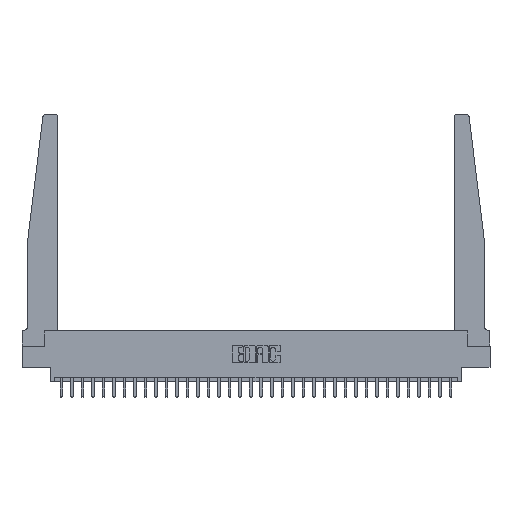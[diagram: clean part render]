
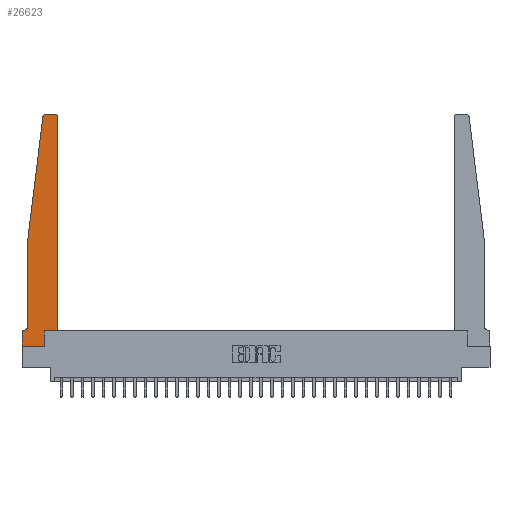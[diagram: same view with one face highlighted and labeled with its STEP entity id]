
A CAD part, top view. The second image highlights one B-rep face of the part: STEP entity #26623.
In plain terms, the highlighted planar face has unit normal (0, 0, 1).
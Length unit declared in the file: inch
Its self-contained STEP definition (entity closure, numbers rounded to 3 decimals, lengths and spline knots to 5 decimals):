
#387 = ORIENTED_EDGE ( 'NONE', *, *, #27444, .T. ) ;
#1822 = VECTOR ( 'NONE', #2126, 39.37008 ) ;
#1898 = CARTESIAN_POINT ( 'NONE',  ( 0.27653, 2.72, 0.37 ) ) ;
#2126 = DIRECTION ( 'NONE',  ( -1., 0., 0. ) ) ;
#2242 = CARTESIAN_POINT ( 'NONE',  ( 0.25, 2.75, 0.37 ) ) ;
#2247 = DIRECTION ( 'NONE',  ( 0., 1., 0. ) ) ;
#2527 = EDGE_CURVE ( 'NONE', #8599, #23406, #13665, .T. ) ;
#2587 = LINE ( 'NONE', #27826, #1822 ) ;
#2915 = EDGE_CURVE ( 'NONE', #23406, #12471, #2587, .T. ) ;
#3376 = VERTEX_POINT ( 'NONE', #18267 ) ;
#4134 = PLANE ( 'NONE',  #16970 ) ;
#4220 = VECTOR ( 'NONE', #27223, 39.37008 ) ;
#4279 = DIRECTION ( 'NONE',  ( 1., 0., 0. ) ) ;
#4394 = DIRECTION ( 'NONE',  ( -0.122, -0.992, 0. ) ) ;
#5062 = LINE ( 'NONE', #23875, #29171 ) ;
#6013 = VERTEX_POINT ( 'NONE', #14080 ) ;
#6069 = VECTOR ( 'NONE', #4394, 39.37008 ) ;
#6763 = AXIS2_PLACEMENT_3D ( 'NONE', #26341, #12355, #28664 ) ;
#6806 = LINE ( 'NONE', #27824, #6069 ) ;
#7369 = VERTEX_POINT ( 'NONE', #12664 ) ;
#7890 = CARTESIAN_POINT ( 'NONE',  ( 0., 0.1875, 0.37 ) ) ;
#8506 = ORIENTED_EDGE ( 'NONE', *, *, #21793, .T. ) ;
#8599 = VERTEX_POINT ( 'NONE', #24033 ) ;
#9480 = CARTESIAN_POINT ( 'NONE',  ( 0.395, 2.72, 0.37 ) ) ;
#10293 = CARTESIAN_POINT ( 'NONE',  ( 0.015, 0.1875, 0.37 ) ) ;
#10484 = EDGE_CURVE ( 'NONE', #17360, #7369, #5062, .T. ) ;
#10695 = AXIS2_PLACEMENT_3D ( 'NONE', #1898, #18375, #4279 ) ;
#10699 = CARTESIAN_POINT ( 'NONE',  ( 0.395, 2.75, 0.37 ) ) ;
#10746 = ORIENTED_EDGE ( 'NONE', *, *, #30219, .T. ) ;
#10862 = CARTESIAN_POINT ( 'NONE',  ( 0.065, 1.25, 0.37 ) ) ;
#11195 = CARTESIAN_POINT ( 'NONE',  ( 0., 0.1875, 0.37 ) ) ;
#11690 = CARTESIAN_POINT ( 'NONE',  ( 0.425, 0.18, 0.37 ) ) ;
#11843 = DIRECTION ( 'NONE',  ( 1., 0., 0. ) ) ;
#12089 = CARTESIAN_POINT ( 'NONE',  ( 0., 0., 0.37 ) ) ;
#12327 = VECTOR ( 'NONE', #2247, 39.37008 ) ;
#12355 = DIRECTION ( 'NONE',  ( 0., 0., -1. ) ) ;
#12471 = VERTEX_POINT ( 'NONE', #7890 ) ;
#12664 = CARTESIAN_POINT ( 'NONE',  ( 0.2605, 0., 0.37 ) ) ;
#13452 = CARTESIAN_POINT ( 'NONE',  ( 0.2605, 0.18, 0.37 ) ) ;
#13602 = DIRECTION ( 'NONE',  ( 1., 0., 0. ) ) ;
#13665 = CIRCLE ( 'NONE', #6763, 0.05 ) ;
#13998 = CARTESIAN_POINT ( 'NONE',  ( 0.2605, 0.18, 0.37 ) ) ;
#14019 = CARTESIAN_POINT ( 'NONE',  ( 0.425, 0.18, 0.37 ) ) ;
#14080 = CARTESIAN_POINT ( 'NONE',  ( 0.24675, 2.72367, 0.37 ) ) ;
#14672 = VECTOR ( 'NONE', #25717, 39.37008 ) ;
#14915 = ORIENTED_EDGE ( 'NONE', *, *, #28834, .T. ) ;
#15337 = VERTEX_POINT ( 'NONE', #27471 ) ;
#15404 = LINE ( 'NONE', #2242, #14672 ) ;
#15406 = DIRECTION ( 'NONE',  ( 0., -1., 0. ) ) ;
#16041 = VECTOR ( 'NONE', #15406, 39.37008 ) ;
#16129 = LINE ( 'NONE', #11690, #21579 ) ;
#16193 = VECTOR ( 'NONE', #27963, 39.37008 ) ;
#16355 = LINE ( 'NONE', #10862, #4220 ) ;
#16633 = EDGE_CURVE ( 'NONE', #26479, #3376, #15404, .T. ) ;
#16970 = AXIS2_PLACEMENT_3D ( 'NONE', #11195, #27553, #13602 ) ;
#17002 = DIRECTION ( 'NONE',  ( 1., 0., 0. ) ) ;
#17360 = VERTEX_POINT ( 'NONE', #12089 ) ;
#17455 = ORIENTED_EDGE ( 'NONE', *, *, #2915, .T. ) ;
#17570 = ORIENTED_EDGE ( 'NONE', *, *, #10484, .T. ) ;
#18267 = CARTESIAN_POINT ( 'NONE',  ( 0.27653, 2.75, 0.37 ) ) ;
#18375 = DIRECTION ( 'NONE',  ( 0., 0., 1. ) ) ;
#18518 = EDGE_CURVE ( 'NONE', #7369, #24363, #18580, .T. ) ;
#18539 = ORIENTED_EDGE ( 'NONE', *, *, #19853, .T. ) ;
#18580 = LINE ( 'NONE', #13998, #12327 ) ;
#19853 = EDGE_CURVE ( 'NONE', #3376, #6013, #22836, .T. ) ;
#21579 = VECTOR ( 'NONE', #28036, 39.37008 ) ;
#21793 = EDGE_CURVE ( 'NONE', #22196, #15337, #28540, .T. ) ;
#22196 = VERTEX_POINT ( 'NONE', #29570 ) ;
#22487 = EDGE_LOOP ( 'NONE', ( #25049, #18539, #10746, #28318, #28690, #17455, #14915, #17570, #29575, #387, #8506, #28704 ) ) ;
#22836 = CIRCLE ( 'NONE', #10695, 0.03 ) ;
#22930 = LINE ( 'NONE', #29324, #16041 ) ;
#23406 = VERTEX_POINT ( 'NONE', #10293 ) ;
#23875 = CARTESIAN_POINT ( 'NONE',  ( 0., 0., 0.37 ) ) ;
#24033 = CARTESIAN_POINT ( 'NONE',  ( 0.065, 0.2375, 0.37 ) ) ;
#24100 = VERTEX_POINT ( 'NONE', #24277 ) ;
#24190 = AXIS2_PLACEMENT_3D ( 'NONE', #9480, #25843, #11843 ) ;
#24277 = CARTESIAN_POINT ( 'NONE',  ( 0.065, 1.25, 0.37 ) ) ;
#24363 = VERTEX_POINT ( 'NONE', #13452 ) ;
#25049 = ORIENTED_EDGE ( 'NONE', *, *, #16633, .T. ) ;
#25717 = DIRECTION ( 'NONE',  ( -1., 0., 0. ) ) ;
#25843 = DIRECTION ( 'NONE',  ( 0., 0., 1. ) ) ;
#26341 = CARTESIAN_POINT ( 'NONE',  ( 0.015, 0.2375, 0.37 ) ) ;
#26426 = FACE_OUTER_BOUND ( 'NONE', #22487, .T. ) ;
#26479 = VERTEX_POINT ( 'NONE', #10699 ) ;
#26623 = ADVANCED_FACE ( 'NONE', ( #26426 ), #4134, .T. ) ;
#27223 = DIRECTION ( 'NONE',  ( 0., -1., 0. ) ) ;
#27444 = EDGE_CURVE ( 'NONE', #24363, #22196, #16129, .T. ) ;
#27471 = CARTESIAN_POINT ( 'NONE',  ( 0.425, 2.72, 0.37 ) ) ;
#27553 = DIRECTION ( 'NONE',  ( 0., 0., 1. ) ) ;
#27824 = CARTESIAN_POINT ( 'NONE',  ( 0.065, 1.25, 0.37 ) ) ;
#27826 = CARTESIAN_POINT ( 'NONE',  ( 0.065, 0.1875, 0.37 ) ) ;
#27963 = DIRECTION ( 'NONE',  ( 0., 1., 0. ) ) ;
#28036 = DIRECTION ( 'NONE',  ( 1., 0., 0. ) ) ;
#28318 = ORIENTED_EDGE ( 'NONE', *, *, #30033, .T. ) ;
#28540 = LINE ( 'NONE', #14019, #16193 ) ;
#28664 = DIRECTION ( 'NONE',  ( -1., 0., 0. ) ) ;
#28690 = ORIENTED_EDGE ( 'NONE', *, *, #2527, .T. ) ;
#28704 = ORIENTED_EDGE ( 'NONE', *, *, #29776, .T. ) ;
#28834 = EDGE_CURVE ( 'NONE', #12471, #17360, #22930, .T. ) ;
#29070 = CIRCLE ( 'NONE', #24190, 0.03 ) ;
#29171 = VECTOR ( 'NONE', #17002, 39.37008 ) ;
#29324 = CARTESIAN_POINT ( 'NONE',  ( 0., 0., 0.37 ) ) ;
#29570 = CARTESIAN_POINT ( 'NONE',  ( 0.425, 0.18, 0.37 ) ) ;
#29575 = ORIENTED_EDGE ( 'NONE', *, *, #18518, .T. ) ;
#29776 = EDGE_CURVE ( 'NONE', #15337, #26479, #29070, .T. ) ;
#30033 = EDGE_CURVE ( 'NONE', #24100, #8599, #16355, .T. ) ;
#30219 = EDGE_CURVE ( 'NONE', #6013, #24100, #6806, .T. ) ;
